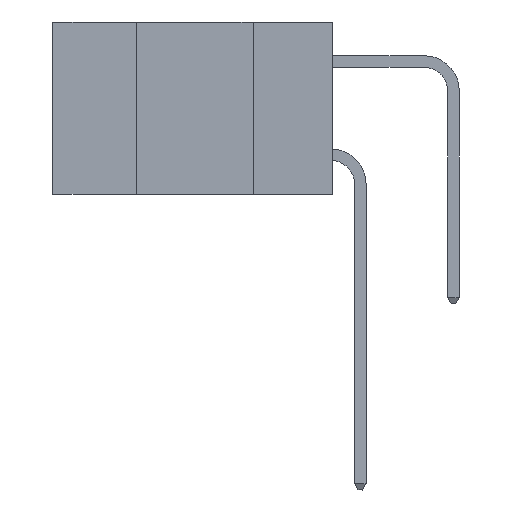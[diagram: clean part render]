
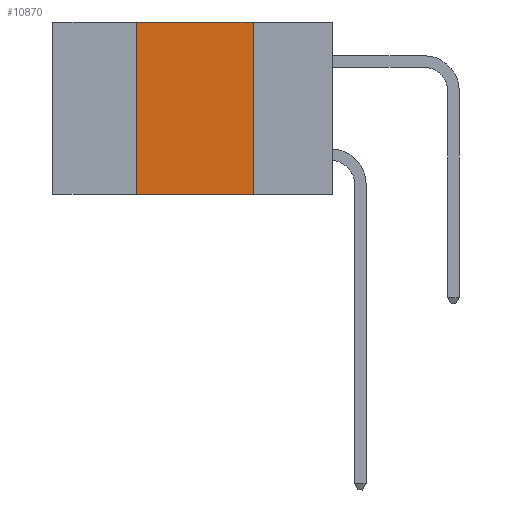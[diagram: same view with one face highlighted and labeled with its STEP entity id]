
A CAD part, left-side view. The second image highlights one B-rep face of the part: STEP entity #10870.
In plain terms, the highlighted planar face has unit normal (-1, 0, 0).
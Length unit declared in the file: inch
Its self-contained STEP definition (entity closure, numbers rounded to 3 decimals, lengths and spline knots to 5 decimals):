
#143 = ORIENTED_EDGE ( 'NONE', *, *, #29138, .F. ) ;
#1004 = VECTOR ( 'NONE', #8206, 39.37008 ) ;
#1221 = VERTEX_POINT ( 'NONE', #25477 ) ;
#2549 = CARTESIAN_POINT ( 'NONE',  ( 0., 0.42, 0. ) ) ;
#3194 = VECTOR ( 'NONE', #13084, 39.37008 ) ;
#6002 = CARTESIAN_POINT ( 'NONE',  ( 0., 0.17, 0. ) ) ;
#6042 = CARTESIAN_POINT ( 'NONE',  ( 0., 0.6, 0. ) ) ;
#6871 = CARTESIAN_POINT ( 'NONE',  ( 0., 0.17, -0.37 ) ) ;
#7020 = VERTEX_POINT ( 'NONE', #6871 ) ;
#8206 = DIRECTION ( 'NONE',  ( 0., 0., 1. ) ) ;
#8212 = ORIENTED_EDGE ( 'NONE', *, *, #12125, .F. ) ;
#8617 = DIRECTION ( 'NONE',  ( 1., 0., 0. ) ) ;
#9026 = DIRECTION ( 'NONE',  ( 0., 0., -1. ) ) ;
#9781 = EDGE_CURVE ( 'NONE', #28366, #7020, #25763, .T. ) ;
#10786 = LINE ( 'NONE', #28390, #3194 ) ;
#10870 = ADVANCED_FACE ( 'NONE', ( #18470 ), #20955, .F. ) ;
#12099 = VECTOR ( 'NONE', #9026, 39.37008 ) ;
#12125 = EDGE_CURVE ( 'NONE', #1221, #14156, #28241, .T. ) ;
#12645 = EDGE_LOOP ( 'NONE', ( #26230, #143, #8212, #17090 ) ) ;
#13084 = DIRECTION ( 'NONE',  ( 0., -1., 0. ) ) ;
#13089 = LINE ( 'NONE', #17711, #32621 ) ;
#14156 = VERTEX_POINT ( 'NONE', #2549 ) ;
#16234 = EDGE_CURVE ( 'NONE', #1221, #7020, #10786, .T. ) ;
#17090 = ORIENTED_EDGE ( 'NONE', *, *, #16234, .T. ) ;
#17711 = CARTESIAN_POINT ( 'NONE',  ( 0., 0.6, 0. ) ) ;
#18470 = FACE_OUTER_BOUND ( 'NONE', #12645, .T. ) ;
#18889 = AXIS2_PLACEMENT_3D ( 'NONE', #6042, #8617, #26559 ) ;
#19344 = CARTESIAN_POINT ( 'NONE',  ( 0., 0.17, 0. ) ) ;
#20304 = DIRECTION ( 'NONE',  ( 0., -1., 0. ) ) ;
#20955 = PLANE ( 'NONE',  #18889 ) ;
#23557 = CARTESIAN_POINT ( 'NONE',  ( 0., 0.42, 0. ) ) ;
#25477 = CARTESIAN_POINT ( 'NONE',  ( 0., 0.42, -0.37 ) ) ;
#25763 = LINE ( 'NONE', #19344, #12099 ) ;
#26230 = ORIENTED_EDGE ( 'NONE', *, *, #9781, .F. ) ;
#26559 = DIRECTION ( 'NONE',  ( 0., 0., -1. ) ) ;
#28241 = LINE ( 'NONE', #23557, #1004 ) ;
#28366 = VERTEX_POINT ( 'NONE', #6002 ) ;
#28390 = CARTESIAN_POINT ( 'NONE',  ( 0., 0.6, -0.37 ) ) ;
#29138 = EDGE_CURVE ( 'NONE', #14156, #28366, #13089, .T. ) ;
#32621 = VECTOR ( 'NONE', #20304, 39.37008 ) ;
